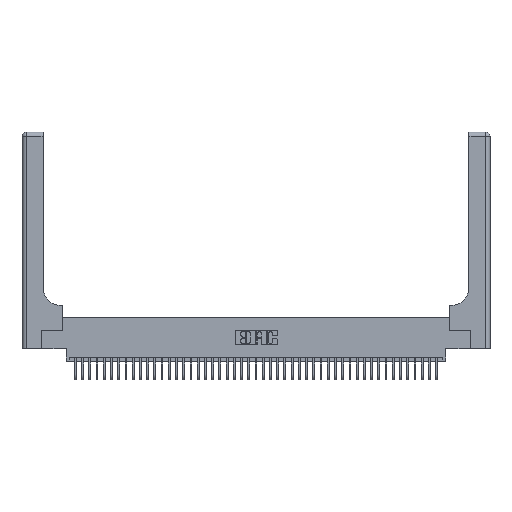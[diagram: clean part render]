
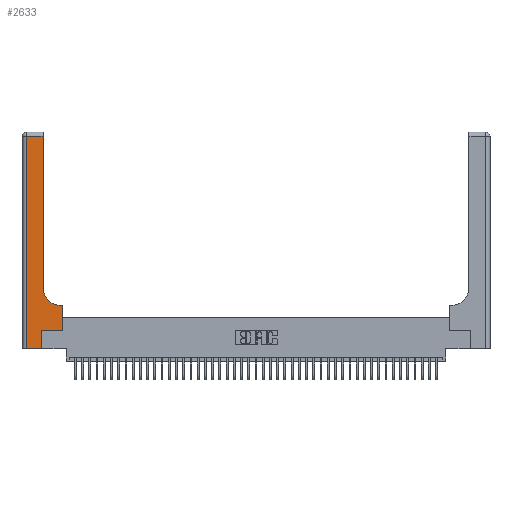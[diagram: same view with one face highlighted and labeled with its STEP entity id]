
A CAD part, top view. The second image highlights one B-rep face of the part: STEP entity #2633.
In plain terms, the highlighted planar face has unit normal (0, 0, 1).
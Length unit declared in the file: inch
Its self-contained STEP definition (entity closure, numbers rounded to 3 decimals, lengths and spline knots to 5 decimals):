
#36 = EDGE_CURVE ( 'NONE', #17804, #33139, #5050, .T. ) ;
#752 = LINE ( 'NONE', #11080, #32843 ) ;
#985 = CARTESIAN_POINT ( 'NONE',  ( 0.5585, 0.25, 0.37 ) ) ;
#1519 = EDGE_CURVE ( 'NONE', #33139, #36287, #35069, .T. ) ;
#1729 = DIRECTION ( 'NONE',  ( -1., 0., 0. ) ) ;
#1864 = VECTOR ( 'NONE', #3849, 39.37008 ) ;
#2633 = ADVANCED_FACE ( 'NONE', ( #12201 ), #43198, .F. ) ;
#3849 = DIRECTION ( 'NONE',  ( 1., 0., 0. ) ) ;
#3923 = DIRECTION ( 'NONE',  ( 1., 0., 0. ) ) ;
#4259 = ORIENTED_EDGE ( 'NONE', *, *, #40412, .T. ) ;
#4264 = LINE ( 'NONE', #9539, #40855 ) ;
#5050 = LINE ( 'NONE', #15630, #13326 ) ;
#5433 = CARTESIAN_POINT ( 'NONE',  ( 0.2915, 2.94, 0.37 ) ) ;
#6298 = DIRECTION ( 'NONE',  ( 0., 1., 0. ) ) ;
#7198 = CARTESIAN_POINT ( 'NONE',  ( 0.2915, 0.85, 0.37 ) ) ;
#9447 = ORIENTED_EDGE ( 'NONE', *, *, #27544, .T. ) ;
#9539 = CARTESIAN_POINT ( 'NONE',  ( 0.5585, 0.25, 0.37 ) ) ;
#9910 = DIRECTION ( 'NONE',  ( 0., 0., -1. ) ) ;
#10919 = CARTESIAN_POINT ( 'NONE',  ( 0.269, 0., 0.37 ) ) ;
#11080 = CARTESIAN_POINT ( 'NONE',  ( 0.2915, 0.6, 0.37 ) ) ;
#11781 = LINE ( 'NONE', #45379, #1864 ) ;
#11816 = DIRECTION ( 'NONE',  ( -1., 0., 0. ) ) ;
#12201 = FACE_OUTER_BOUND ( 'NONE', #21690, .T. ) ;
#13326 = VECTOR ( 'NONE', #1729, 39.37008 ) ;
#13923 = ORIENTED_EDGE ( 'NONE', *, *, #27518, .T. ) ;
#14168 = CARTESIAN_POINT ( 'NONE',  ( 0.06, 2.94, 0.37 ) ) ;
#14520 = ORIENTED_EDGE ( 'NONE', *, *, #40641, .T. ) ;
#15630 = CARTESIAN_POINT ( 'NONE',  ( 0., 2.94, 0.37 ) ) ;
#16186 = VECTOR ( 'NONE', #26114, 39.37008 ) ;
#16755 = CARTESIAN_POINT ( 'NONE',  ( 0.269, 0.25, 0.37 ) ) ;
#17305 = LINE ( 'NONE', #18148, #20051 ) ;
#17496 = LINE ( 'NONE', #39524, #21932 ) ;
#17804 = VERTEX_POINT ( 'NONE', #5433 ) ;
#18148 = CARTESIAN_POINT ( 'NONE',  ( 0.269, 0., 0.37 ) ) ;
#18338 = ORIENTED_EDGE ( 'NONE', *, *, #18399, .T. ) ;
#18399 = EDGE_CURVE ( 'NONE', #43868, #17804, #44584, .T. ) ;
#19774 = DIRECTION ( 'NONE',  ( 0., 1., 0. ) ) ;
#20051 = VECTOR ( 'NONE', #42998, 39.37008 ) ;
#20083 = CARTESIAN_POINT ( 'NONE',  ( 0.2915, 3., 0.37 ) ) ;
#21500 = AXIS2_PLACEMENT_3D ( 'NONE', #42400, #9910, #31575 ) ;
#21690 = EDGE_LOOP ( 'NONE', ( #18338, #43768, #32316, #14520, #9447, #13923, #4259, #25102, #28939 ) ) ;
#21932 = VECTOR ( 'NONE', #3923, 39.37008 ) ;
#22955 = VERTEX_POINT ( 'NONE', #16755 ) ;
#23455 = VERTEX_POINT ( 'NONE', #24880 ) ;
#24880 = CARTESIAN_POINT ( 'NONE',  ( 0.5585, 0.6, 0.37 ) ) ;
#24961 = VERTEX_POINT ( 'NONE', #985 ) ;
#25102 = ORIENTED_EDGE ( 'NONE', *, *, #27605, .T. ) ;
#26114 = DIRECTION ( 'NONE',  ( 0., -1., 0. ) ) ;
#26504 = CARTESIAN_POINT ( 'NONE',  ( 0.5415, 0.6, 0.37 ) ) ;
#27456 = EDGE_CURVE ( 'NONE', #28594, #43868, #40067, .T. ) ;
#27518 = EDGE_CURVE ( 'NONE', #22955, #24961, #11781, .T. ) ;
#27544 = EDGE_CURVE ( 'NONE', #43255, #22955, #17305, .T. ) ;
#27605 = EDGE_CURVE ( 'NONE', #23455, #28594, #752, .T. ) ;
#28594 = VERTEX_POINT ( 'NONE', #26504 ) ;
#28939 = ORIENTED_EDGE ( 'NONE', *, *, #27456, .T. ) ;
#28997 = VECTOR ( 'NONE', #19774, 39.37008 ) ;
#29223 = CARTESIAN_POINT ( 'NONE',  ( 0.06, 3., 0.37 ) ) ;
#30931 = CARTESIAN_POINT ( 'NONE',  ( 0.06, 0., 0.37 ) ) ;
#31575 = DIRECTION ( 'NONE',  ( 1., 0., 0. ) ) ;
#32316 = ORIENTED_EDGE ( 'NONE', *, *, #1519, .T. ) ;
#32843 = VECTOR ( 'NONE', #39599, 39.37008 ) ;
#33038 = DIRECTION ( 'NONE',  ( 0., 0., -1. ) ) ;
#33139 = VERTEX_POINT ( 'NONE', #14168 ) ;
#34067 = CARTESIAN_POINT ( 'NONE',  ( 0., 3., 0.37 ) ) ;
#35069 = LINE ( 'NONE', #29223, #16186 ) ;
#36287 = VERTEX_POINT ( 'NONE', #30931 ) ;
#39524 = CARTESIAN_POINT ( 'NONE',  ( 0., 0., 0.37 ) ) ;
#39599 = DIRECTION ( 'NONE',  ( -1., 0., 0. ) ) ;
#40067 = CIRCLE ( 'NONE', #21500, 0.25 ) ;
#40412 = EDGE_CURVE ( 'NONE', #24961, #23455, #4264, .T. ) ;
#40641 = EDGE_CURVE ( 'NONE', #36287, #43255, #17496, .T. ) ;
#40855 = VECTOR ( 'NONE', #6298, 39.37008 ) ;
#41442 = AXIS2_PLACEMENT_3D ( 'NONE', #34067, #33038, #11816 ) ;
#42400 = CARTESIAN_POINT ( 'NONE',  ( 0.5415, 0.85, 0.37 ) ) ;
#42998 = DIRECTION ( 'NONE',  ( 0., 1., 0. ) ) ;
#43198 = PLANE ( 'NONE',  #41442 ) ;
#43255 = VERTEX_POINT ( 'NONE', #10919 ) ;
#43768 = ORIENTED_EDGE ( 'NONE', *, *, #36, .T. ) ;
#43868 = VERTEX_POINT ( 'NONE', #7198 ) ;
#44584 = LINE ( 'NONE', #20083, #28997 ) ;
#45379 = CARTESIAN_POINT ( 'NONE',  ( 0.269, 0.25, 0.37 ) ) ;
